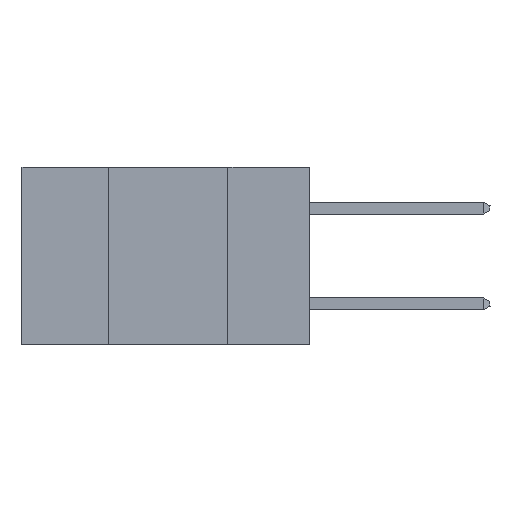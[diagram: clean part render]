
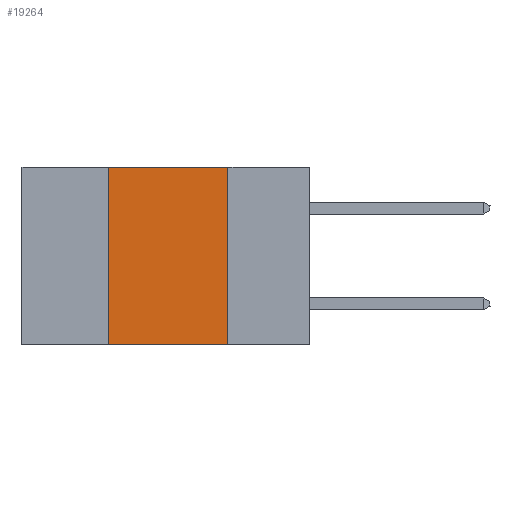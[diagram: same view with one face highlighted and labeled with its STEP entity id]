
A CAD part, left-side view. The second image highlights one B-rep face of the part: STEP entity #19264.
In plain terms, the highlighted planar face has unit normal (-1, 0, 0).
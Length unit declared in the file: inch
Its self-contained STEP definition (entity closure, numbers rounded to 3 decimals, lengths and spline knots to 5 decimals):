
#1260 = CARTESIAN_POINT ( 'NONE',  ( 0., 0.6, 0. ) ) ;
#1756 = CARTESIAN_POINT ( 'NONE',  ( 0., 0.42, 0. ) ) ;
#2046 = ORIENTED_EDGE ( 'NONE', *, *, #25499, .F. ) ;
#2684 = CARTESIAN_POINT ( 'NONE',  ( 0., 0.17, 0. ) ) ;
#2873 = EDGE_LOOP ( 'NONE', ( #32168, #16677, #2046, #15648 ) ) ;
#3565 = FACE_OUTER_BOUND ( 'NONE', #2873, .T. ) ;
#3644 = AXIS2_PLACEMENT_3D ( 'NONE', #1260, #36758, #33501 ) ;
#6079 = VERTEX_POINT ( 'NONE', #8822 ) ;
#8675 = VECTOR ( 'NONE', #31793, 39.37008 ) ;
#8822 = CARTESIAN_POINT ( 'NONE',  ( 0., 0.42, -0.37 ) ) ;
#10364 = DIRECTION ( 'NONE',  ( 0., 0., -1. ) ) ;
#10615 = CARTESIAN_POINT ( 'NONE',  ( 0., 0.6, -0.37 ) ) ;
#12798 = LINE ( 'NONE', #10615, #8675 ) ;
#13240 = LINE ( 'NONE', #25770, #14178 ) ;
#13697 = DIRECTION ( 'NONE',  ( 0., 0., 1. ) ) ;
#14178 = VECTOR ( 'NONE', #19937, 39.37008 ) ;
#15648 = ORIENTED_EDGE ( 'NONE', *, *, #37553, .T. ) ;
#15790 = CARTESIAN_POINT ( 'NONE',  ( 0., 0.42, 0. ) ) ;
#16677 = ORIENTED_EDGE ( 'NONE', *, *, #34296, .F. ) ;
#19264 = ADVANCED_FACE ( 'NONE', ( #3565 ), #21747, .F. ) ;
#19937 = DIRECTION ( 'NONE',  ( 0., -1., 0. ) ) ;
#20757 = VECTOR ( 'NONE', #10364, 39.37008 ) ;
#20879 = VERTEX_POINT ( 'NONE', #37423 ) ;
#21747 = PLANE ( 'NONE',  #3644 ) ;
#22487 = CARTESIAN_POINT ( 'NONE',  ( 0., 0.17, 0. ) ) ;
#25499 = EDGE_CURVE ( 'NONE', #6079, #27736, #37228, .T. ) ;
#25770 = CARTESIAN_POINT ( 'NONE',  ( 0., 0.6, 0. ) ) ;
#27465 = VERTEX_POINT ( 'NONE', #2684 ) ;
#27736 = VERTEX_POINT ( 'NONE', #15790 ) ;
#28895 = EDGE_CURVE ( 'NONE', #27465, #20879, #34625, .T. ) ;
#31793 = DIRECTION ( 'NONE',  ( 0., -1., 0. ) ) ;
#32168 = ORIENTED_EDGE ( 'NONE', *, *, #28895, .F. ) ;
#33501 = DIRECTION ( 'NONE',  ( 0., 0., -1. ) ) ;
#34296 = EDGE_CURVE ( 'NONE', #27736, #27465, #13240, .T. ) ;
#34625 = LINE ( 'NONE', #22487, #20757 ) ;
#36758 = DIRECTION ( 'NONE',  ( 1., 0., 0. ) ) ;
#36784 = VECTOR ( 'NONE', #13697, 39.37008 ) ;
#37228 = LINE ( 'NONE', #1756, #36784 ) ;
#37423 = CARTESIAN_POINT ( 'NONE',  ( 0., 0.17, -0.37 ) ) ;
#37553 = EDGE_CURVE ( 'NONE', #6079, #20879, #12798, .T. ) ;
